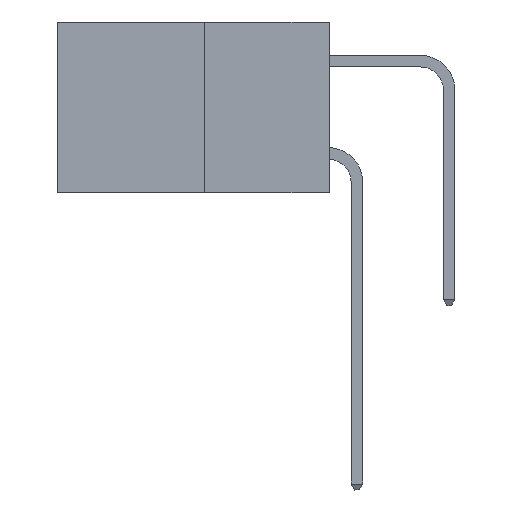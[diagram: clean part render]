
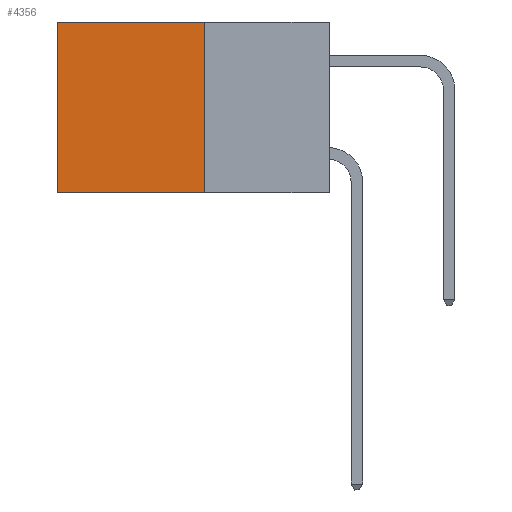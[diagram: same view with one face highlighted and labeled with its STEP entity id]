
A CAD part, left-side view. The second image highlights one B-rep face of the part: STEP entity #4356.
In plain terms, the highlighted planar face has unit normal (-1, 0, 0).
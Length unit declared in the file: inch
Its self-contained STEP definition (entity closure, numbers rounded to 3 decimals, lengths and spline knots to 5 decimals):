
#692 = EDGE_CURVE ( 'NONE', #21716, #14986, #17137, .T. ) ;
#2067 = LINE ( 'NONE', #19804, #16663 ) ;
#2728 = ORIENTED_EDGE ( 'NONE', *, *, #6749, .F. ) ;
#3012 = ORIENTED_EDGE ( 'NONE', *, *, #12917, .F. ) ;
#4356 = ADVANCED_FACE ( 'NONE', ( #5214 ), #13390, .F. ) ;
#4914 = VERTEX_POINT ( 'NONE', #13025 ) ;
#5214 = FACE_OUTER_BOUND ( 'NONE', #21547, .T. ) ;
#5689 = DIRECTION ( 'NONE',  ( 0., 0., -1. ) ) ;
#5708 = CARTESIAN_POINT ( 'NONE',  ( 0.277, 0.27, 0. ) ) ;
#6251 = VECTOR ( 'NONE', #23312, 39.37008 ) ;
#6749 = EDGE_CURVE ( 'NONE', #21716, #8031, #11420, .T. ) ;
#7110 = VECTOR ( 'NONE', #5689, 39.37008 ) ;
#7829 = CARTESIAN_POINT ( 'NONE',  ( 0.277, 0.27, 0. ) ) ;
#8031 = VERTEX_POINT ( 'NONE', #13011 ) ;
#8176 = ORIENTED_EDGE ( 'NONE', *, *, #692, .T. ) ;
#9133 = VECTOR ( 'NONE', #14446, 39.37008 ) ;
#10471 = ORIENTED_EDGE ( 'NONE', *, *, #10822, .T. ) ;
#10822 = EDGE_CURVE ( 'NONE', #14986, #4914, #2067, .T. ) ;
#11147 = CARTESIAN_POINT ( 'NONE',  ( 0.277, 0.27, -0.37 ) ) ;
#11420 = LINE ( 'NONE', #11147, #7110 ) ;
#12572 = DIRECTION ( 'NONE',  ( 0., 0., -1. ) ) ;
#12917 = EDGE_CURVE ( 'NONE', #8031, #4914, #15153, .T. ) ;
#13011 = CARTESIAN_POINT ( 'NONE',  ( 0.277, 0.27, -0.37 ) ) ;
#13025 = CARTESIAN_POINT ( 'NONE',  ( 0.277, 0.59, -0.37 ) ) ;
#13180 = DIRECTION ( 'NONE',  ( 0., 0., -1. ) ) ;
#13313 = DIRECTION ( 'NONE',  ( 1., 0., 0. ) ) ;
#13390 = PLANE ( 'NONE',  #17808 ) ;
#14134 = CARTESIAN_POINT ( 'NONE',  ( 0.277, 0.27, -0.37 ) ) ;
#14446 = DIRECTION ( 'NONE',  ( 0., 1., 0. ) ) ;
#14986 = VERTEX_POINT ( 'NONE', #16530 ) ;
#15153 = LINE ( 'NONE', #19851, #9133 ) ;
#16530 = CARTESIAN_POINT ( 'NONE',  ( 0.277, 0.59, 0. ) ) ;
#16663 = VECTOR ( 'NONE', #12572, 39.37008 ) ;
#17137 = LINE ( 'NONE', #5708, #6251 ) ;
#17808 = AXIS2_PLACEMENT_3D ( 'NONE', #14134, #13313, #13180 ) ;
#19804 = CARTESIAN_POINT ( 'NONE',  ( 0.277, 0.59, -0.37 ) ) ;
#19851 = CARTESIAN_POINT ( 'NONE',  ( 0.277, 0.27, -0.37 ) ) ;
#21547 = EDGE_LOOP ( 'NONE', ( #10471, #3012, #2728, #8176 ) ) ;
#21716 = VERTEX_POINT ( 'NONE', #7829 ) ;
#23312 = DIRECTION ( 'NONE',  ( 0., 1., 0. ) ) ;
